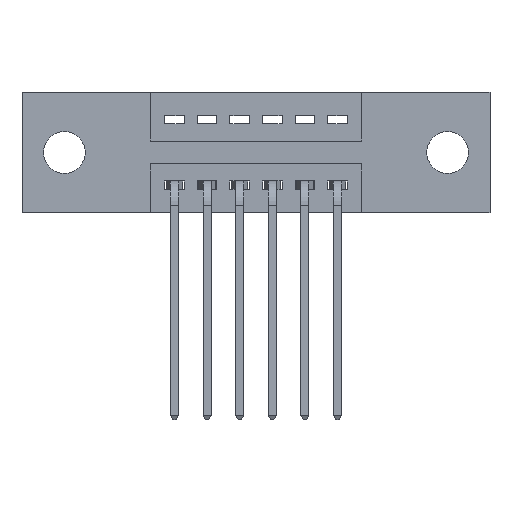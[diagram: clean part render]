
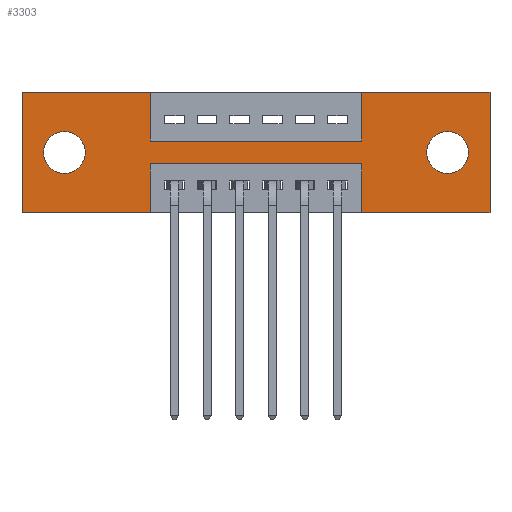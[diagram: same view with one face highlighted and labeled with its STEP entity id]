
A CAD part, front view. The second image highlights one B-rep face of the part: STEP entity #3303.
In plain terms, the highlighted planar face has unit normal (0, -1, 0).
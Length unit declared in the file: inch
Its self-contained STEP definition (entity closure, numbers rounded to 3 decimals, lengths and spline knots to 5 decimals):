
#42 = DIRECTION ( 'NONE',  ( 0., 0., 1. ) ) ;
#107 = CARTESIAN_POINT ( 'NONE',  ( 0.13, 0., -0.185 ) ) ;
#127 = VECTOR ( 'NONE', #7327, 39.37008 ) ;
#129 = EDGE_CURVE ( 'NONE', #6463, #8581, #5758, .T. ) ;
#140 = DIRECTION ( 'NONE',  ( 1., 0., 0. ) ) ;
#176 = DIRECTION ( 'NONE',  ( 0., 1., 0. ) ) ;
#192 = DIRECTION ( 'NONE',  ( 0., 0., 1. ) ) ;
#220 = CARTESIAN_POINT ( 'NONE',  ( 0.3925, 0., -0.37 ) ) ;
#224 = AXIS2_PLACEMENT_3D ( 'NONE', #107, #176, #5236 ) ;
#241 = VERTEX_POINT ( 'NONE', #8379 ) ;
#256 = ORIENTED_EDGE ( 'NONE', *, *, #1791, .T. ) ;
#306 = CARTESIAN_POINT ( 'NONE',  ( 0., 0., 0. ) ) ;
#320 = CARTESIAN_POINT ( 'NONE',  ( 0., 0., -0.37 ) ) ;
#337 = CARTESIAN_POINT ( 'NONE',  ( 1.305, 0., -0.249 ) ) ;
#421 = EDGE_CURVE ( 'NONE', #4975, #6463, #6045, .T. ) ;
#554 = CARTESIAN_POINT ( 'NONE',  ( 0., 0., 0. ) ) ;
#648 = LINE ( 'NONE', #320, #4308 ) ;
#701 = LINE ( 'NONE', #2130, #2412 ) ;
#747 = DIRECTION ( 'NONE',  ( 0., 0., -1. ) ) ;
#870 = CIRCLE ( 'NONE', #6958, 0.064 ) ;
#895 = EDGE_CURVE ( 'NONE', #4334, #1366, #870, .T. ) ;
#1226 = VECTOR ( 'NONE', #2490, 39.37008 ) ;
#1264 = VERTEX_POINT ( 'NONE', #220 ) ;
#1281 = EDGE_CURVE ( 'NONE', #1264, #241, #648, .T. ) ;
#1322 = CARTESIAN_POINT ( 'NONE',  ( 1.435, 0., 0. ) ) ;
#1366 = VERTEX_POINT ( 'NONE', #2628 ) ;
#1380 = FACE_BOUND ( 'NONE', #8705, .T. ) ;
#1529 = VECTOR ( 'NONE', #3426, 39.37008 ) ;
#1634 = EDGE_CURVE ( 'NONE', #8349, #7263, #5113, .T. ) ;
#1657 = DIRECTION ( 'NONE',  ( -1., 0., 0. ) ) ;
#1771 = EDGE_LOOP ( 'NONE', ( #6926, #3300 ) ) ;
#1791 = EDGE_CURVE ( 'NONE', #1366, #4334, #2228, .T. ) ;
#1909 = EDGE_CURVE ( 'NONE', #2363, #6226, #1970, .T. ) ;
#1941 = FACE_BOUND ( 'NONE', #1771, .T. ) ;
#1970 = LINE ( 'NONE', #6100, #8962 ) ;
#2130 = CARTESIAN_POINT ( 'NONE',  ( 0., 0., 0. ) ) ;
#2228 = CIRCLE ( 'NONE', #224, 0.064 ) ;
#2268 = CARTESIAN_POINT ( 'NONE',  ( 0.13, 0., -0.121 ) ) ;
#2294 = DIRECTION ( 'NONE',  ( 0., 0., 1. ) ) ;
#2328 = ORIENTED_EDGE ( 'NONE', *, *, #3561, .F. ) ;
#2350 = CARTESIAN_POINT ( 'NONE',  ( 1.0425, 0., -0.37 ) ) ;
#2363 = VERTEX_POINT ( 'NONE', #8841 ) ;
#2412 = VECTOR ( 'NONE', #140, 39.37008 ) ;
#2486 = CARTESIAN_POINT ( 'NONE',  ( 0.13, 0., -0.185 ) ) ;
#2490 = DIRECTION ( 'NONE',  ( 0., 0., -1. ) ) ;
#2497 = VERTEX_POINT ( 'NONE', #8861 ) ;
#2567 = VERTEX_POINT ( 'NONE', #9042 ) ;
#2628 = CARTESIAN_POINT ( 'NONE',  ( 0.13, 0., -0.249 ) ) ;
#2916 = CARTESIAN_POINT ( 'NONE',  ( 0., 0., -0.37 ) ) ;
#3231 = AXIS2_PLACEMENT_3D ( 'NONE', #9458, #7968, #8733 ) ;
#3284 = CARTESIAN_POINT ( 'NONE',  ( 0.3925, 0., 0. ) ) ;
#3300 = ORIENTED_EDGE ( 'NONE', *, *, #6632, .T. ) ;
#3303 = ADVANCED_FACE ( 'NONE', ( #1941, #1380, #7818 ), #6584, .T. ) ;
#3353 = CIRCLE ( 'NONE', #5281, 0.064 ) ;
#3418 = EDGE_CURVE ( 'NONE', #241, #8349, #4268, .T. ) ;
#3426 = DIRECTION ( 'NONE',  ( 1., 0., 0. ) ) ;
#3561 = EDGE_CURVE ( 'NONE', #3707, #4975, #701, .T. ) ;
#3707 = VERTEX_POINT ( 'NONE', #4203 ) ;
#3729 = ORIENTED_EDGE ( 'NONE', *, *, #5888, .F. ) ;
#3862 = CARTESIAN_POINT ( 'NONE',  ( 1.435, 0., 0. ) ) ;
#3975 = EDGE_CURVE ( 'NONE', #2567, #1264, #8811, .T. ) ;
#4058 = ORIENTED_EDGE ( 'NONE', *, *, #421, .F. ) ;
#4203 = CARTESIAN_POINT ( 'NONE',  ( 1.0425, 0., 0. ) ) ;
#4244 = CARTESIAN_POINT ( 'NONE',  ( 0.3925, 0., -0.37 ) ) ;
#4268 = LINE ( 'NONE', #7303, #7929 ) ;
#4308 = VECTOR ( 'NONE', #6119, 39.37008 ) ;
#4334 = VERTEX_POINT ( 'NONE', #2268 ) ;
#4558 = LINE ( 'NONE', #5293, #7087 ) ;
#4975 = VERTEX_POINT ( 'NONE', #3862 ) ;
#5113 = LINE ( 'NONE', #554, #1529 ) ;
#5146 = ORIENTED_EDGE ( 'NONE', *, *, #895, .T. ) ;
#5172 = EDGE_CURVE ( 'NONE', #7263, #2363, #9002, .T. ) ;
#5179 = CARTESIAN_POINT ( 'NONE',  ( 1.0425, 0., -0.15 ) ) ;
#5236 = DIRECTION ( 'NONE',  ( 0., 0., 1. ) ) ;
#5281 = AXIS2_PLACEMENT_3D ( 'NONE', #6714, #6012, #8130 ) ;
#5293 = CARTESIAN_POINT ( 'NONE',  ( 1.0425, 0., -0.37 ) ) ;
#5315 = ORIENTED_EDGE ( 'NONE', *, *, #1909, .F. ) ;
#5409 = ORIENTED_EDGE ( 'NONE', *, *, #129, .F. ) ;
#5523 = DIRECTION ( 'NONE',  ( 0., 1., 0. ) ) ;
#5706 = ORIENTED_EDGE ( 'NONE', *, *, #8319, .F. ) ;
#5758 = LINE ( 'NONE', #8974, #8373 ) ;
#5841 = VERTEX_POINT ( 'NONE', #6545 ) ;
#5888 = EDGE_CURVE ( 'NONE', #8581, #2497, #4558, .T. ) ;
#6012 = DIRECTION ( 'NONE',  ( 0., 1., 0. ) ) ;
#6045 = LINE ( 'NONE', #1322, #8422 ) ;
#6100 = CARTESIAN_POINT ( 'NONE',  ( 0.3925, 0., -0.15 ) ) ;
#6119 = DIRECTION ( 'NONE',  ( -1., 0., 0. ) ) ;
#6226 = VERTEX_POINT ( 'NONE', #5179 ) ;
#6403 = ORIENTED_EDGE ( 'NONE', *, *, #3418, .F. ) ;
#6463 = VERTEX_POINT ( 'NONE', #9172 ) ;
#6545 = CARTESIAN_POINT ( 'NONE',  ( 1.305, 0., -0.121 ) ) ;
#6584 = PLANE ( 'NONE',  #7892 ) ;
#6632 = EDGE_CURVE ( 'NONE', #8759, #5841, #7640, .T. ) ;
#6714 = CARTESIAN_POINT ( 'NONE',  ( 1.305, 0., -0.185 ) ) ;
#6805 = CARTESIAN_POINT ( 'NONE',  ( 0.3925, 0., 0. ) ) ;
#6889 = CARTESIAN_POINT ( 'NONE',  ( 0.3925, 0., -0.22 ) ) ;
#6924 = VECTOR ( 'NONE', #1657, 39.37008 ) ;
#6926 = ORIENTED_EDGE ( 'NONE', *, *, #7128, .T. ) ;
#6958 = AXIS2_PLACEMENT_3D ( 'NONE', #2486, #5523, #8458 ) ;
#6964 = DIRECTION ( 'NONE',  ( 1., 0., 0. ) ) ;
#7041 = LINE ( 'NONE', #6889, #6924 ) ;
#7087 = VECTOR ( 'NONE', #2294, 39.37008 ) ;
#7098 = ORIENTED_EDGE ( 'NONE', *, *, #1281, .F. ) ;
#7128 = EDGE_CURVE ( 'NONE', #5841, #8759, #3353, .T. ) ;
#7263 = VERTEX_POINT ( 'NONE', #6805 ) ;
#7273 = DIRECTION ( 'NONE',  ( 0., -1., 0. ) ) ;
#7303 = CARTESIAN_POINT ( 'NONE',  ( 0., 0., 0. ) ) ;
#7327 = DIRECTION ( 'NONE',  ( 0., 0., -1. ) ) ;
#7352 = ORIENTED_EDGE ( 'NONE', *, *, #5172, .F. ) ;
#7461 = EDGE_LOOP ( 'NONE', ( #9099, #5706, #3729, #5409, #4058, #2328, #8236, #5315, #7352, #7558, #6403, #7098 ) ) ;
#7558 = ORIENTED_EDGE ( 'NONE', *, *, #1634, .F. ) ;
#7640 = CIRCLE ( 'NONE', #3231, 0.064 ) ;
#7818 = FACE_OUTER_BOUND ( 'NONE', #7461, .T. ) ;
#7892 = AXIS2_PLACEMENT_3D ( 'NONE', #2916, #7273, #747 ) ;
#7911 = DIRECTION ( 'NONE',  ( 0., 0., -1. ) ) ;
#7929 = VECTOR ( 'NONE', #42, 39.37008 ) ;
#7968 = DIRECTION ( 'NONE',  ( 0., 1., 0. ) ) ;
#8130 = DIRECTION ( 'NONE',  ( 0., 0., -1. ) ) ;
#8236 = ORIENTED_EDGE ( 'NONE', *, *, #8399, .F. ) ;
#8319 = EDGE_CURVE ( 'NONE', #2497, #2567, #7041, .T. ) ;
#8349 = VERTEX_POINT ( 'NONE', #306 ) ;
#8373 = VECTOR ( 'NONE', #9132, 39.37008 ) ;
#8379 = CARTESIAN_POINT ( 'NONE',  ( 0., 0., -0.37 ) ) ;
#8388 = LINE ( 'NONE', #8895, #8729 ) ;
#8399 = EDGE_CURVE ( 'NONE', #6226, #3707, #8388, .T. ) ;
#8422 = VECTOR ( 'NONE', #7911, 39.37008 ) ;
#8458 = DIRECTION ( 'NONE',  ( 0., 0., 1. ) ) ;
#8581 = VERTEX_POINT ( 'NONE', #2350 ) ;
#8705 = EDGE_LOOP ( 'NONE', ( #5146, #256 ) ) ;
#8729 = VECTOR ( 'NONE', #192, 39.37008 ) ;
#8733 = DIRECTION ( 'NONE',  ( 0., 0., -1. ) ) ;
#8759 = VERTEX_POINT ( 'NONE', #337 ) ;
#8811 = LINE ( 'NONE', #4244, #127 ) ;
#8841 = CARTESIAN_POINT ( 'NONE',  ( 0.3925, 0., -0.15 ) ) ;
#8861 = CARTESIAN_POINT ( 'NONE',  ( 1.0425, 0., -0.22 ) ) ;
#8895 = CARTESIAN_POINT ( 'NONE',  ( 1.0425, 0., 0. ) ) ;
#8962 = VECTOR ( 'NONE', #6964, 39.37008 ) ;
#8974 = CARTESIAN_POINT ( 'NONE',  ( 0., 0., -0.37 ) ) ;
#9002 = LINE ( 'NONE', #3284, #1226 ) ;
#9042 = CARTESIAN_POINT ( 'NONE',  ( 0.3925, 0., -0.22 ) ) ;
#9099 = ORIENTED_EDGE ( 'NONE', *, *, #3975, .F. ) ;
#9132 = DIRECTION ( 'NONE',  ( -1., 0., 0. ) ) ;
#9172 = CARTESIAN_POINT ( 'NONE',  ( 1.435, 0., -0.37 ) ) ;
#9458 = CARTESIAN_POINT ( 'NONE',  ( 1.305, 0., -0.185 ) ) ;
